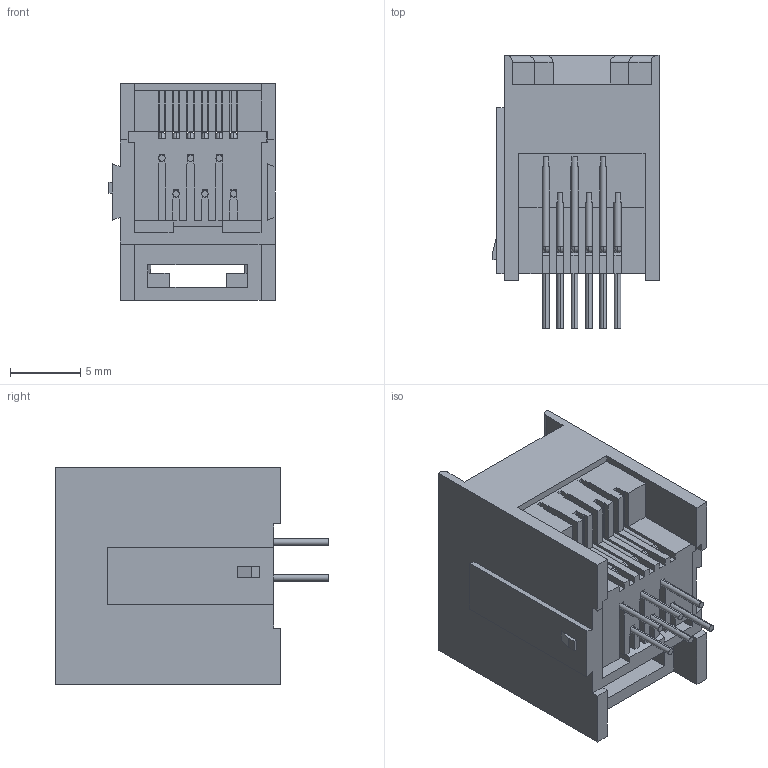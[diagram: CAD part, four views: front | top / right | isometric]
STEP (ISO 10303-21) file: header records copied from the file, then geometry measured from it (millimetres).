
FILE_DESCRIPTION (( 'STEP AP203' ), '1' );
FILE_NAME ('J2X016691P00030.STEP', '2020-07-29T15:00:48', ( '' ), ( '' ), 'SwSTEP 2.0', 'SolidWorks 2020', '' );
FILE_SCHEMA (( 'CONFIG_CONTROL_DESIGN' ));
Length unit declared in the file: millimetre
Products named in the file (4): 2X Contacts_6P6C; J2X016691P00030; 2X Insulator; 2X Contact Lock
Assembly tree (3 placements, depth 2):
  J2X016691P00030
    2X Insulator
    2X Contacts_6P6C
    2X Contact Lock
Bounding box: 11.81 x 19.4 x 15.4 mm (x, y, z)
Volume: 1218.6 mm3; surface area: 2843.8 mm2
Topology: 8 solids, 8 shells, 466 faces, 1369 edges, 877 vertices
Faces by surface type: plane 333, cylinder 97, bspline 36
Entity records: 16612 total; most frequent: CARTESIAN_POINT 3903, ORIENTED_EDGE 2690, DIRECTION 2447, EDGE_CURVE 1345, VECTOR 1075, LINE 1075, VERTEX_POINT 877, AXIS2_PLACEMENT_3D 686
